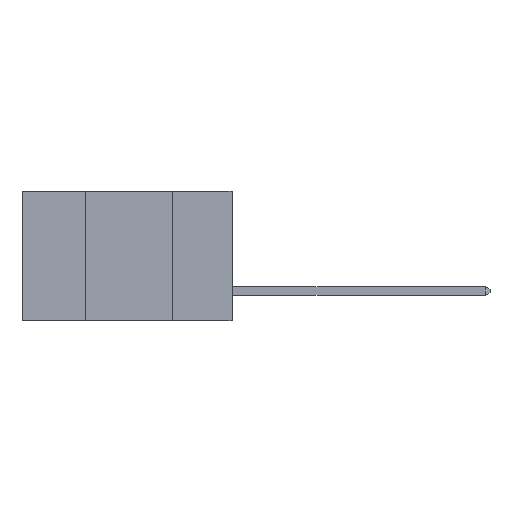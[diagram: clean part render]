
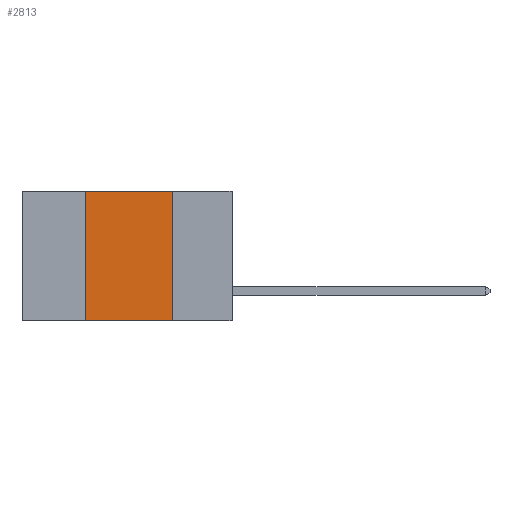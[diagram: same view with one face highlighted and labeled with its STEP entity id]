
A CAD part, left-side view. The second image highlights one B-rep face of the part: STEP entity #2813.
In plain terms, the highlighted planar face has unit normal (-1, 0, 0).
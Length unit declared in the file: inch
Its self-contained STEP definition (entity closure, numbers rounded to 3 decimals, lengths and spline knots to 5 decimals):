
#1225 = PLANE ( 'NONE',  #2549 ) ;
#2021 = CARTESIAN_POINT ( 'NONE',  ( 0., 0.42, 0. ) ) ;
#2314 = EDGE_CURVE ( 'NONE', #7896, #2321, #5056, .T. ) ;
#2321 = VERTEX_POINT ( 'NONE', #8110 ) ;
#2473 = VECTOR ( 'NONE', #11810, 39.37008 ) ;
#2549 = AXIS2_PLACEMENT_3D ( 'NONE', #6766, #6780, #12061 ) ;
#2582 = CARTESIAN_POINT ( 'NONE',  ( 0., 0.17, 0. ) ) ;
#2789 = EDGE_CURVE ( 'NONE', #8716, #2321, #5040, .T. ) ;
#2813 = ADVANCED_FACE ( 'NONE', ( #9681 ), #1225, .F. ) ;
#3459 = EDGE_LOOP ( 'NONE', ( #6475, #4524, #10827, #6982 ) ) ;
#3771 = DIRECTION ( 'NONE',  ( 0., 0., -1. ) ) ;
#4524 = ORIENTED_EDGE ( 'NONE', *, *, #5227, .F. ) ;
#5040 = LINE ( 'NONE', #7514, #12593 ) ;
#5056 = LINE ( 'NONE', #2582, #7303 ) ;
#5086 = VERTEX_POINT ( 'NONE', #2021 ) ;
#5227 = EDGE_CURVE ( 'NONE', #5086, #7896, #9426, .T. ) ;
#6475 = ORIENTED_EDGE ( 'NONE', *, *, #2314, .F. ) ;
#6699 = VECTOR ( 'NONE', #10872, 39.37008 ) ;
#6750 = CARTESIAN_POINT ( 'NONE',  ( 0., 0.42, 0. ) ) ;
#6766 = CARTESIAN_POINT ( 'NONE',  ( 0., 0.6, 0. ) ) ;
#6780 = DIRECTION ( 'NONE',  ( 1., 0., 0. ) ) ;
#6799 = CARTESIAN_POINT ( 'NONE',  ( 0., 0.42, -0.37 ) ) ;
#6982 = ORIENTED_EDGE ( 'NONE', *, *, #2789, .T. ) ;
#7303 = VECTOR ( 'NONE', #3771, 39.37008 ) ;
#7514 = CARTESIAN_POINT ( 'NONE',  ( 0., 0.6, -0.37 ) ) ;
#7896 = VERTEX_POINT ( 'NONE', #8489 ) ;
#8110 = CARTESIAN_POINT ( 'NONE',  ( 0., 0.17, -0.37 ) ) ;
#8489 = CARTESIAN_POINT ( 'NONE',  ( 0., 0.17, 0. ) ) ;
#8674 = EDGE_CURVE ( 'NONE', #8716, #5086, #13557, .T. ) ;
#8716 = VERTEX_POINT ( 'NONE', #6799 ) ;
#9426 = LINE ( 'NONE', #11474, #6699 ) ;
#9681 = FACE_OUTER_BOUND ( 'NONE', #3459, .T. ) ;
#10113 = DIRECTION ( 'NONE',  ( 0., -1., 0. ) ) ;
#10827 = ORIENTED_EDGE ( 'NONE', *, *, #8674, .F. ) ;
#10872 = DIRECTION ( 'NONE',  ( 0., -1., 0. ) ) ;
#11474 = CARTESIAN_POINT ( 'NONE',  ( 0., 0.6, 0. ) ) ;
#11810 = DIRECTION ( 'NONE',  ( 0., 0., 1. ) ) ;
#12061 = DIRECTION ( 'NONE',  ( 0., 0., -1. ) ) ;
#12593 = VECTOR ( 'NONE', #10113, 39.37008 ) ;
#13557 = LINE ( 'NONE', #6750, #2473 ) ;
